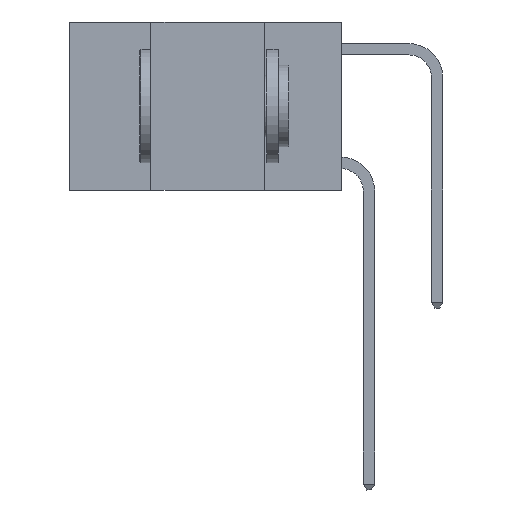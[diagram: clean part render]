
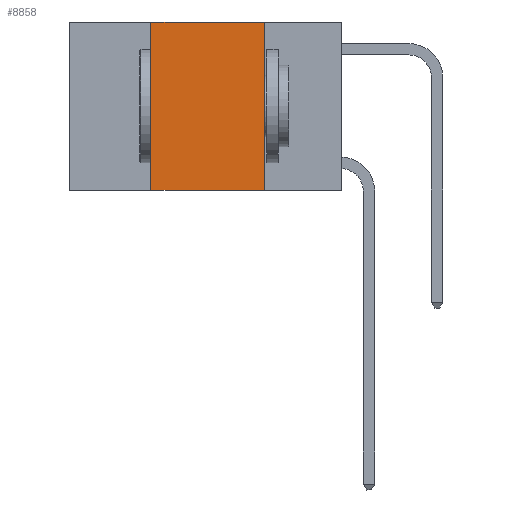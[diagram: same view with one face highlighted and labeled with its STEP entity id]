
A CAD part, left-side view. The second image highlights one B-rep face of the part: STEP entity #8858.
In plain terms, the highlighted planar face has unit normal (-1, 0, 0).
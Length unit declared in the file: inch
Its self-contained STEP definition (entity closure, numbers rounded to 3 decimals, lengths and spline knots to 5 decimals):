
#103 = VERTEX_POINT ( 'NONE', #11121 ) ;
#152 = VERTEX_POINT ( 'NONE', #4855 ) ;
#567 = VERTEX_POINT ( 'NONE', #7568 ) ;
#634 = EDGE_CURVE ( 'NONE', #152, #7008, #5496, .T. ) ;
#861 = FACE_OUTER_BOUND ( 'NONE', #4568, .T. ) ;
#876 = CARTESIAN_POINT ( 'NONE',  ( 0., 0.6, 0. ) ) ;
#1221 = PLANE ( 'NONE',  #6855 ) ;
#1268 = VECTOR ( 'NONE', #8130, 39.37008 ) ;
#1306 = EDGE_CURVE ( 'NONE', #103, #567, #10227, .T. ) ;
#1661 = VECTOR ( 'NONE', #5594, 39.37008 ) ;
#2411 = ORIENTED_EDGE ( 'NONE', *, *, #1306, .T. ) ;
#2779 = EDGE_CURVE ( 'NONE', #7008, #567, #10192, .T. ) ;
#2988 = CARTESIAN_POINT ( 'NONE',  ( 0., 0.6, 0. ) ) ;
#3577 = VECTOR ( 'NONE', #7325, 39.37008 ) ;
#4192 = CARTESIAN_POINT ( 'NONE',  ( 0., 0.17, 0. ) ) ;
#4389 = ORIENTED_EDGE ( 'NONE', *, *, #2779, .F. ) ;
#4568 = EDGE_LOOP ( 'NONE', ( #4389, #11039, #10458, #2411 ) ) ;
#4855 = CARTESIAN_POINT ( 'NONE',  ( 0., 0.42, 0. ) ) ;
#5408 = DIRECTION ( 'NONE',  ( 0., -1., 0. ) ) ;
#5496 = LINE ( 'NONE', #876, #10103 ) ;
#5585 = DIRECTION ( 'NONE',  ( 0., 0., -1. ) ) ;
#5594 = DIRECTION ( 'NONE',  ( 0., 0., 1. ) ) ;
#5934 = CARTESIAN_POINT ( 'NONE',  ( 0., 0.17, 0. ) ) ;
#6800 = LINE ( 'NONE', #10770, #1661 ) ;
#6855 = AXIS2_PLACEMENT_3D ( 'NONE', #2988, #10765, #5585 ) ;
#7008 = VERTEX_POINT ( 'NONE', #5934 ) ;
#7325 = DIRECTION ( 'NONE',  ( 0., 0., -1. ) ) ;
#7568 = CARTESIAN_POINT ( 'NONE',  ( 0., 0.17, -0.37 ) ) ;
#8130 = DIRECTION ( 'NONE',  ( 0., -1., 0. ) ) ;
#8858 = ADVANCED_FACE ( 'NONE', ( #861 ), #1221, .F. ) ;
#8924 = CARTESIAN_POINT ( 'NONE',  ( 0., 0.6, -0.37 ) ) ;
#10098 = EDGE_CURVE ( 'NONE', #103, #152, #6800, .T. ) ;
#10103 = VECTOR ( 'NONE', #5408, 39.37008 ) ;
#10192 = LINE ( 'NONE', #4192, #3577 ) ;
#10227 = LINE ( 'NONE', #8924, #1268 ) ;
#10458 = ORIENTED_EDGE ( 'NONE', *, *, #10098, .F. ) ;
#10765 = DIRECTION ( 'NONE',  ( 1., 0., 0. ) ) ;
#10770 = CARTESIAN_POINT ( 'NONE',  ( 0., 0.42, 0. ) ) ;
#11039 = ORIENTED_EDGE ( 'NONE', *, *, #634, .F. ) ;
#11121 = CARTESIAN_POINT ( 'NONE',  ( 0., 0.42, -0.37 ) ) ;
